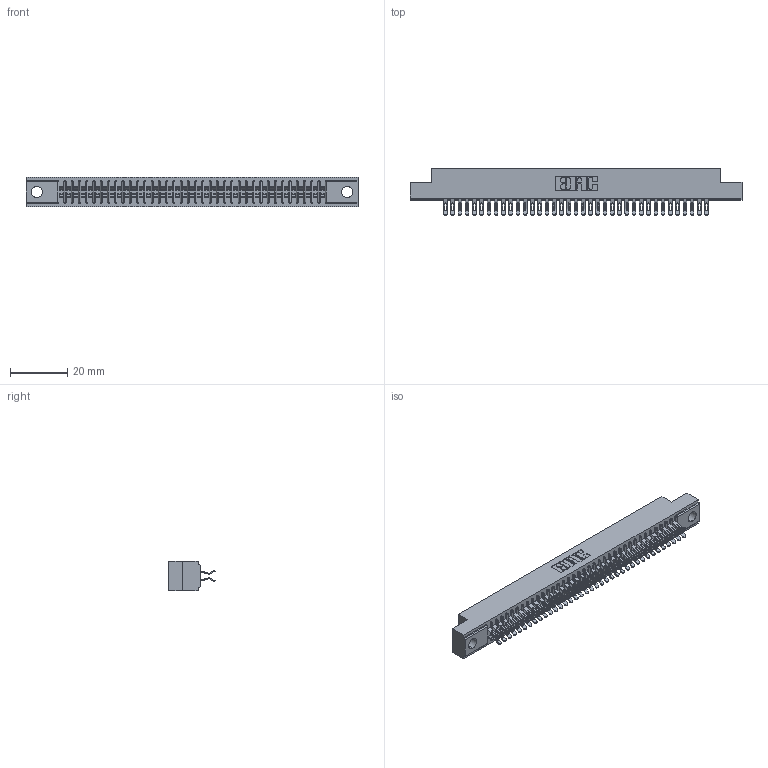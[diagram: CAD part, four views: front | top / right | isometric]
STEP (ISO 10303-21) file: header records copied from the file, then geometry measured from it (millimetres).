
FILE_DESCRIPTION (( 'STEP AP203' ), '1' );
FILE_NAME ('391-074-555-204.STEP', '2018-08-09T14:45:29', ( '' ), ( '' ), 'SwSTEP 2.0', 'SolidWorks 2016', '' );
FILE_SCHEMA (( 'CONFIG_CONTROL_DESIGN' ));
Length unit declared in the file: inch
Products named in the file (3): 341-292-001_341-292-155; 391-074-555-204; 341 Part_.156 (3.96) Dia Mounting Holes
Assembly tree (75 placements, depth 2):
  391-074-555-204
    341 Part_.156 (3.96) Dia Mounting Holes
    341-292-001_341-292-155  x74
Bounding box: 116.2 x 16.31 x 10.16 mm (x, y, z)
Volume: 8564.8 mm3; surface area: 15536.2 mm2
Topology: 75 solids, 75 shells, 5902 faces, 17631 edges, 11478 vertices
Faces by surface type: plane 3190, cylinder 2564, sphere 76, torus 72
Entity records: 46332 total; most frequent: CARTESIAN_POINT 7723, ORIENTED_EDGE 7662, DIRECTION 7481, EDGE_CURVE 3831, LINE 3081, VECTOR 3081, VERTEX_POINT 2426, AXIS2_PLACEMENT_3D 2200
